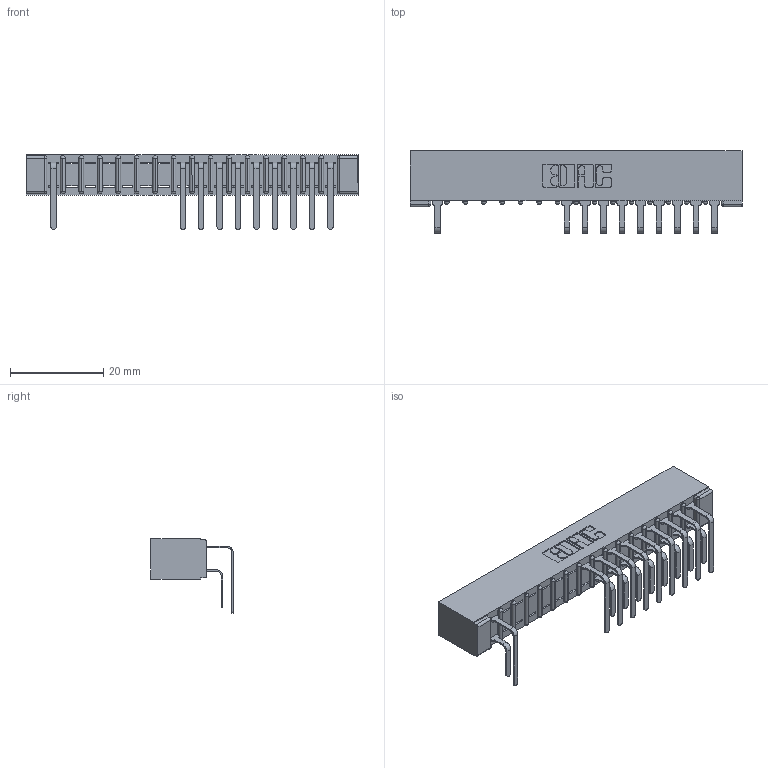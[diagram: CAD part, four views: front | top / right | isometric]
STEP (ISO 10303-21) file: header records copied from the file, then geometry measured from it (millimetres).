
FILE_DESCRIPTION (( 'STEP AP203' ), '1' );
FILE_NAME ('307-032-559-201.STEP', '2018-08-04T22:55:06', ( '' ), ( '' ), 'SwSTEP 2.0', 'SolidWorks 2016', '' );
FILE_SCHEMA (( 'CONFIG_CONTROL_DESIGN' ));
Length unit declared in the file: inch
Products named in the file (4): 307 Part_No Mounting Lugs; 307-290-001_558 559 - 1 (Single); 307-290-001_559 - 2 (Single); 307-032-559-201
Assembly tree (20 placements, depth 2):
  307-032-559-201
    307 Part_No Mounting Lugs
    307-290-001_558 559 - 1 (Single)  x9
    307-290-001_559 - 2 (Single)  x10
Bounding box: 71.27 x 17.69 x 16.08 mm (x, y, z)
Volume: 4813.3 mm3; surface area: 8149.4 mm2
Topology: 20 solids, 20 shells, 1207 faces, 3413 edges, 2202 vertices
Faces by surface type: plane 771, cylinder 402, sphere 34
Entity records: 18187 total; most frequent: CARTESIAN_POINT 3037, ORIENTED_EDGE 3018, DIRECTION 2971, EDGE_CURVE 1509, VECTOR 1147, LINE 1147, VERTEX_POINT 978, AXIS2_PLACEMENT_3D 912
